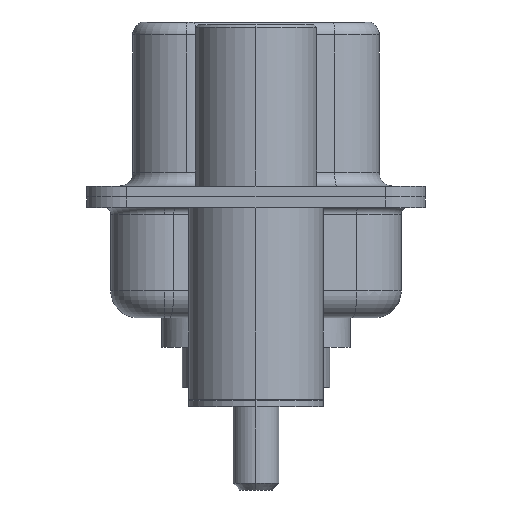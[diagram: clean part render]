
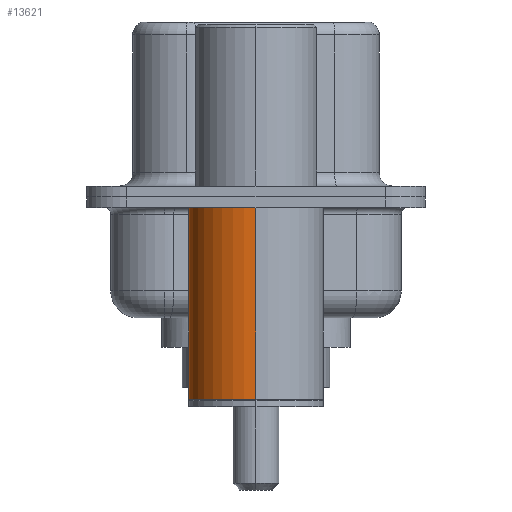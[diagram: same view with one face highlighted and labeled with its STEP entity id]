
A CAD part, left-side view. The second image highlights one B-rep face of the part: STEP entity #13621.
In plain terms, the highlighted cylindrical face has radius 2.5 mm (diameter 5 mm), a partial arc.
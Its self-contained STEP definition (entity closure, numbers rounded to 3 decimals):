
#1031 = AXIS2_PLACEMENT_3D ( 'NONE', #7540, #16132, #8809 ) ;
#1157 = CARTESIAN_POINT ( 'NONE',  ( 2.5, 0., -7.525 ) ) ;
#1220 = CARTESIAN_POINT ( 'NONE',  ( 0., 0., -0.4 ) ) ;
#1382 = ORIENTED_EDGE ( 'NONE', *, *, #11491, .T. ) ;
#1820 = ORIENTED_EDGE ( 'NONE', *, *, #12156, .F. ) ;
#1942 = DIRECTION ( 'NONE',  ( 0., 0., 1. ) ) ;
#1968 = EDGE_CURVE ( 'NONE', #2045, #13799, #12504, .T. ) ;
#2045 = VERTEX_POINT ( 'NONE', #1157 ) ;
#2555 = DIRECTION ( 'NONE',  ( 1., 0., 0. ) ) ;
#2764 = ORIENTED_EDGE ( 'NONE', *, *, #5413, .F. ) ;
#3034 = LINE ( 'NONE', #13964, #15398 ) ;
#3103 = ORIENTED_EDGE ( 'NONE', *, *, #1968, .T. ) ;
#3194 = FACE_OUTER_BOUND ( 'NONE', #10423, .T. ) ;
#4115 = CIRCLE ( 'NONE', #4238, 2.5 ) ;
#4238 = AXIS2_PLACEMENT_3D ( 'NONE', #1220, #10042, #2555 ) ;
#5413 = EDGE_CURVE ( 'NONE', #15911, #6109, #4115, .T. ) ;
#5479 = LINE ( 'NONE', #15558, #15009 ) ;
#5569 = CARTESIAN_POINT ( 'NONE',  ( 0., 0., 0.581 ) ) ;
#6109 = VERTEX_POINT ( 'NONE', #13774 ) ;
#7540 = CARTESIAN_POINT ( 'NONE',  ( 0., 0., -7.525 ) ) ;
#8356 = AXIS2_PLACEMENT_3D ( 'NONE', #5569, #9428, #13008 ) ;
#8809 = DIRECTION ( 'NONE',  ( 1., 0., 0. ) ) ;
#9428 = DIRECTION ( 'NONE',  ( 0., 0., 1. ) ) ;
#9456 = CYLINDRICAL_SURFACE ( 'NONE', #8356, 2.5 ) ;
#10042 = DIRECTION ( 'NONE',  ( 0., 0., 1. ) ) ;
#10321 = DIRECTION ( 'NONE',  ( 0., 0., 1. ) ) ;
#10423 = EDGE_LOOP ( 'NONE', ( #3103, #1382, #2764, #1820 ) ) ;
#11491 = EDGE_CURVE ( 'NONE', #13799, #6109, #3034, .T. ) ;
#12156 = EDGE_CURVE ( 'NONE', #2045, #15911, #5479, .T. ) ;
#12504 = CIRCLE ( 'NONE', #1031, 2.5 ) ;
#13008 = DIRECTION ( 'NONE',  ( 1., 0., 0. ) ) ;
#13621 = ADVANCED_FACE ( 'NONE', ( #3194 ), #9456, .T. ) ;
#13774 = CARTESIAN_POINT ( 'NONE',  ( -2.5, 0., -0.4 ) ) ;
#13799 = VERTEX_POINT ( 'NONE', #15943 ) ;
#13964 = CARTESIAN_POINT ( 'NONE',  ( -2.5, 0., 0.581 ) ) ;
#13995 = CARTESIAN_POINT ( 'NONE',  ( 2.5, 0., -0.4 ) ) ;
#15009 = VECTOR ( 'NONE', #1942, 1000. ) ;
#15398 = VECTOR ( 'NONE', #10321, 1000. ) ;
#15558 = CARTESIAN_POINT ( 'NONE',  ( 2.5, 0., 0.581 ) ) ;
#15911 = VERTEX_POINT ( 'NONE', #13995 ) ;
#15943 = CARTESIAN_POINT ( 'NONE',  ( -2.5, 0., -7.525 ) ) ;
#16132 = DIRECTION ( 'NONE',  ( 0., 0., 1. ) ) ;
